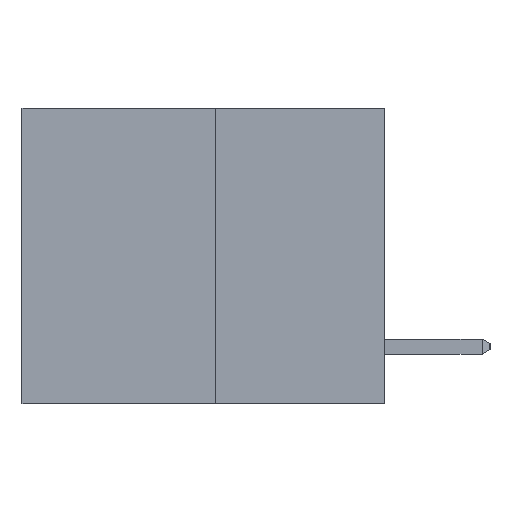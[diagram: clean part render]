
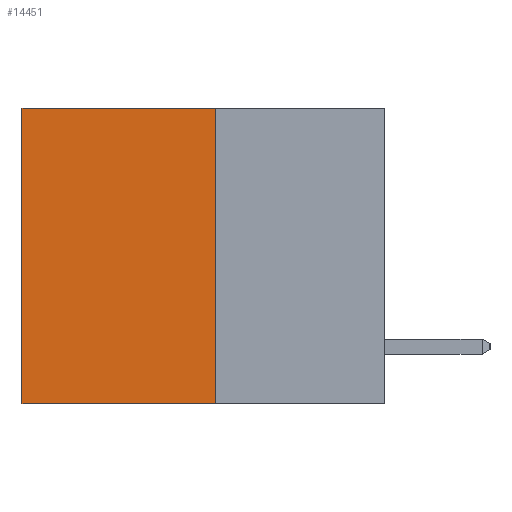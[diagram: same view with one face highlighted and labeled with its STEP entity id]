
A CAD part, left-side view. The second image highlights one B-rep face of the part: STEP entity #14451.
In plain terms, the highlighted planar face has unit normal (-1, 0, 0).
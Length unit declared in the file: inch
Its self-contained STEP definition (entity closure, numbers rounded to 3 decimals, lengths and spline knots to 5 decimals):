
#953 = DIRECTION ( 'NONE',  ( 0., 0., -1. ) ) ;
#1555 = VECTOR ( 'NONE', #14640, 39.37008 ) ;
#1624 = CARTESIAN_POINT ( 'NONE',  ( 0.3165, 0.6, -0.49 ) ) ;
#1743 = LINE ( 'NONE', #17703, #4108 ) ;
#2492 = VERTEX_POINT ( 'NONE', #15515 ) ;
#2643 = AXIS2_PLACEMENT_3D ( 'NONE', #6134, #8927, #15849 ) ;
#3476 = ORIENTED_EDGE ( 'NONE', *, *, #5169, .T. ) ;
#3725 = DIRECTION ( 'NONE',  ( 0., 1., 0. ) ) ;
#3772 = CARTESIAN_POINT ( 'NONE',  ( 0.3165, 0.28, 0. ) ) ;
#4108 = VECTOR ( 'NONE', #3725, 39.37008 ) ;
#4121 = EDGE_LOOP ( 'NONE', ( #3476, #9907, #16473, #9301 ) ) ;
#4380 = LINE ( 'NONE', #12100, #9623 ) ;
#5169 = EDGE_CURVE ( 'NONE', #8168, #6910, #8505, .T. ) ;
#6134 = CARTESIAN_POINT ( 'NONE',  ( 0.3165, 0.28, -0.49 ) ) ;
#6910 = VERTEX_POINT ( 'NONE', #17014 ) ;
#7494 = CARTESIAN_POINT ( 'NONE',  ( 0.3165, 0.6, 0. ) ) ;
#8168 = VERTEX_POINT ( 'NONE', #7494 ) ;
#8505 = LINE ( 'NONE', #1624, #10885 ) ;
#8767 = CARTESIAN_POINT ( 'NONE',  ( 0.3165, 0.28, -0.49 ) ) ;
#8927 = DIRECTION ( 'NONE',  ( 1., 0., 0. ) ) ;
#9223 = EDGE_CURVE ( 'NONE', #16644, #2492, #4380, .T. ) ;
#9301 = ORIENTED_EDGE ( 'NONE', *, *, #11234, .T. ) ;
#9516 = FACE_OUTER_BOUND ( 'NONE', #4121, .T. ) ;
#9623 = VECTOR ( 'NONE', #953, 39.37008 ) ;
#9766 = DIRECTION ( 'NONE',  ( 0., 0., -1. ) ) ;
#9907 = ORIENTED_EDGE ( 'NONE', *, *, #16246, .F. ) ;
#10885 = VECTOR ( 'NONE', #9766, 39.37008 ) ;
#11234 = EDGE_CURVE ( 'NONE', #16644, #8168, #1743, .T. ) ;
#12100 = CARTESIAN_POINT ( 'NONE',  ( 0.3165, 0.28, -0.49 ) ) ;
#13043 = PLANE ( 'NONE',  #2643 ) ;
#14451 = ADVANCED_FACE ( 'NONE', ( #9516 ), #13043, .F. ) ;
#14640 = DIRECTION ( 'NONE',  ( 0., 1., 0. ) ) ;
#15515 = CARTESIAN_POINT ( 'NONE',  ( 0.3165, 0.28, -0.49 ) ) ;
#15849 = DIRECTION ( 'NONE',  ( 0., 0., -1. ) ) ;
#16246 = EDGE_CURVE ( 'NONE', #2492, #6910, #17622, .T. ) ;
#16473 = ORIENTED_EDGE ( 'NONE', *, *, #9223, .F. ) ;
#16644 = VERTEX_POINT ( 'NONE', #3772 ) ;
#17014 = CARTESIAN_POINT ( 'NONE',  ( 0.3165, 0.6, -0.49 ) ) ;
#17622 = LINE ( 'NONE', #8767, #1555 ) ;
#17703 = CARTESIAN_POINT ( 'NONE',  ( 0.3165, 0.28, 0. ) ) ;
